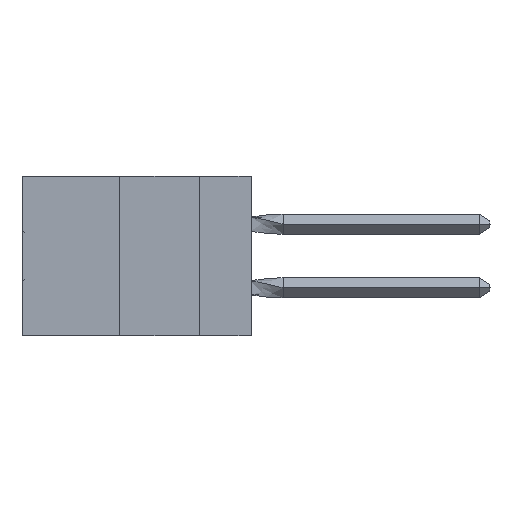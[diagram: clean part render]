
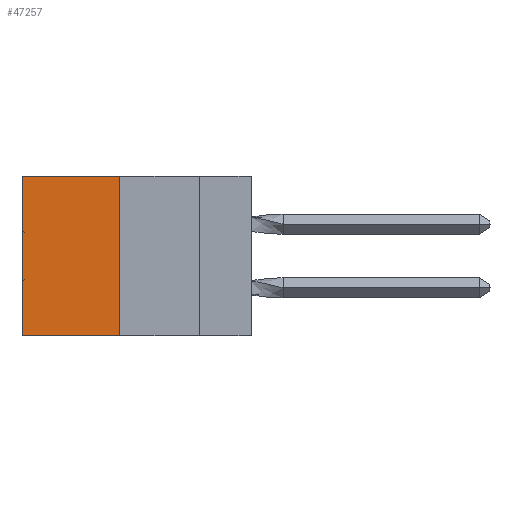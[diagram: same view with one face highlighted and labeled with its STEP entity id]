
A CAD part, left-side view. The second image highlights one B-rep face of the part: STEP entity #47257.
In plain terms, the highlighted planar face has unit normal (-1, 0, 0).
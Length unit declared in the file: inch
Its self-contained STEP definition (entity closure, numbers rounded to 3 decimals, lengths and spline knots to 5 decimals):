
#1662 = VECTOR ( 'NONE', #22692, 39.37008 ) ;
#4419 = VECTOR ( 'NONE', #34033, 39.37008 ) ;
#4968 = EDGE_LOOP ( 'NONE', ( #45364, #18068, #43032, #14994 ) ) ;
#7531 = CARTESIAN_POINT ( 'NONE',  ( 0.305, 0.413, 0. ) ) ;
#7595 = CARTESIAN_POINT ( 'NONE',  ( 0.305, 0.413, -0.5 ) ) ;
#9305 = VERTEX_POINT ( 'NONE', #19584 ) ;
#13819 = AXIS2_PLACEMENT_3D ( 'NONE', #43466, #36168, #24555 ) ;
#14542 = LINE ( 'NONE', #7595, #4419 ) ;
#14947 = CARTESIAN_POINT ( 'NONE',  ( 0.305, 0.72, -0.5 ) ) ;
#14994 = ORIENTED_EDGE ( 'NONE', *, *, #34444, .T. ) ;
#16213 = DIRECTION ( 'NONE',  ( 0., 0., -1. ) ) ;
#16936 = PLANE ( 'NONE',  #13819 ) ;
#18068 = ORIENTED_EDGE ( 'NONE', *, *, #24248, .F. ) ;
#19502 = CARTESIAN_POINT ( 'NONE',  ( 0.305, 0.72, 0. ) ) ;
#19584 = CARTESIAN_POINT ( 'NONE',  ( 0.305, 0.413, -0.5 ) ) ;
#21238 = VERTEX_POINT ( 'NONE', #46161 ) ;
#22692 = DIRECTION ( 'NONE',  ( 0., 1., 0. ) ) ;
#24248 = EDGE_CURVE ( 'NONE', #9305, #30464, #47141, .T. ) ;
#24334 = CARTESIAN_POINT ( 'NONE',  ( 0.305, 0.72, -0.5 ) ) ;
#24555 = DIRECTION ( 'NONE',  ( 0., 0., -1. ) ) ;
#26964 = LINE ( 'NONE', #24334, #34671 ) ;
#29552 = EDGE_CURVE ( 'NONE', #21238, #9305, #14542, .T. ) ;
#30464 = VERTEX_POINT ( 'NONE', #14947 ) ;
#31121 = FACE_OUTER_BOUND ( 'NONE', #4968, .T. ) ;
#31880 = LINE ( 'NONE', #7531, #1662 ) ;
#34033 = DIRECTION ( 'NONE',  ( 0., 0., -1. ) ) ;
#34444 = EDGE_CURVE ( 'NONE', #21238, #48317, #31880, .T. ) ;
#34671 = VECTOR ( 'NONE', #16213, 39.37008 ) ;
#35654 = CARTESIAN_POINT ( 'NONE',  ( 0.305, 0.413, -0.5 ) ) ;
#36168 = DIRECTION ( 'NONE',  ( 1., 0., 0. ) ) ;
#37047 = VECTOR ( 'NONE', #39139, 39.37008 ) ;
#39139 = DIRECTION ( 'NONE',  ( 0., 1., 0. ) ) ;
#43032 = ORIENTED_EDGE ( 'NONE', *, *, #29552, .F. ) ;
#43466 = CARTESIAN_POINT ( 'NONE',  ( 0.305, 0.413, -0.5 ) ) ;
#45364 = ORIENTED_EDGE ( 'NONE', *, *, #47724, .T. ) ;
#46161 = CARTESIAN_POINT ( 'NONE',  ( 0.305, 0.413, 0. ) ) ;
#47141 = LINE ( 'NONE', #35654, #37047 ) ;
#47257 = ADVANCED_FACE ( 'NONE', ( #31121 ), #16936, .F. ) ;
#47724 = EDGE_CURVE ( 'NONE', #48317, #30464, #26964, .T. ) ;
#48317 = VERTEX_POINT ( 'NONE', #19502 ) ;
